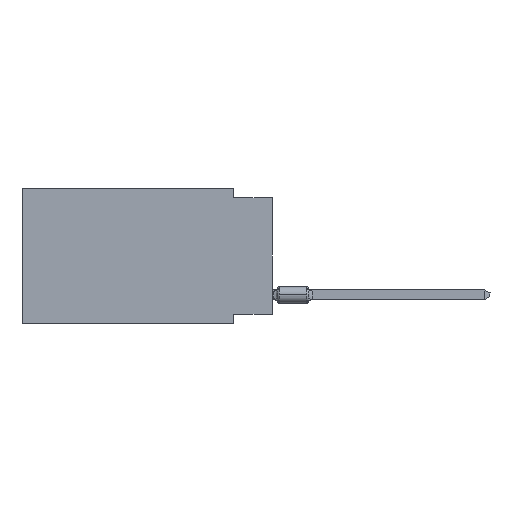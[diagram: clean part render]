
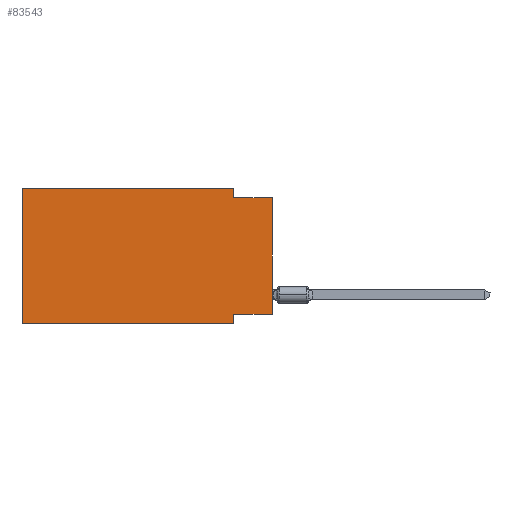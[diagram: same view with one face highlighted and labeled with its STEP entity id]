
A CAD part, left-side view. The second image highlights one B-rep face of the part: STEP entity #83543.
In plain terms, the highlighted planar face has unit normal (-1, 0, 0).
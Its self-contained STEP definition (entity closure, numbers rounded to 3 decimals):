
#1387 = FACE_OUTER_BOUND ( 'NONE', #75346, .T. ) ;
#3332 = DIRECTION ( 'NONE',  ( 0., 0., 1. ) ) ;
#4005 = ORIENTED_EDGE ( 'NONE', *, *, #35180, .F. ) ;
#4529 = CARTESIAN_POINT ( 'NONE',  ( 0., 2.54, -8.89 ) ) ;
#7326 = VERTEX_POINT ( 'NONE', #96517 ) ;
#8008 = CARTESIAN_POINT ( 'NONE',  ( 0., 2.54, -8.89 ) ) ;
#8583 = CARTESIAN_POINT ( 'NONE',  ( 0., 0., -8.255 ) ) ;
#10677 = DIRECTION ( 'NONE',  ( 0., -1., 0. ) ) ;
#14866 = VERTEX_POINT ( 'NONE', #88078 ) ;
#14873 = LINE ( 'NONE', #96654, #21799 ) ;
#15118 = ORIENTED_EDGE ( 'NONE', *, *, #36795, .T. ) ;
#15277 = VERTEX_POINT ( 'NONE', #24820 ) ;
#15380 = CARTESIAN_POINT ( 'NONE',  ( 0., 2.54, 0. ) ) ;
#17217 = DIRECTION ( 'NONE',  ( 0., -1., 0. ) ) ;
#20809 = CARTESIAN_POINT ( 'NONE',  ( 0., 0., -0.635 ) ) ;
#21293 = LINE ( 'NONE', #15380, #52518 ) ;
#21799 = VECTOR ( 'NONE', #104650, 1000. ) ;
#24820 = CARTESIAN_POINT ( 'NONE',  ( 0., 16.383, 0. ) ) ;
#25246 = VECTOR ( 'NONE', #25396, 1000. ) ;
#25396 = DIRECTION ( 'NONE',  ( 0., -1., 0. ) ) ;
#25451 = DIRECTION ( 'NONE',  ( 1., 0., 0. ) ) ;
#35180 = EDGE_CURVE ( 'NONE', #55034, #45108, #90320, .T. ) ;
#35359 = ORIENTED_EDGE ( 'NONE', *, *, #64687, .F. ) ;
#36795 = EDGE_CURVE ( 'NONE', #14866, #80378, #14873, .T. ) ;
#37780 = VECTOR ( 'NONE', #56697, 1000. ) ;
#40611 = DIRECTION ( 'NONE',  ( 0., 0., -1. ) ) ;
#40931 = ORIENTED_EDGE ( 'NONE', *, *, #84051, .F. ) ;
#41956 = LINE ( 'NONE', #49446, #25246 ) ;
#43768 = VECTOR ( 'NONE', #40611, 1000. ) ;
#43943 = LINE ( 'NONE', #76568, #55681 ) ;
#44126 = CARTESIAN_POINT ( 'NONE',  ( 0., 2.54, -8.255 ) ) ;
#44241 = ORIENTED_EDGE ( 'NONE', *, *, #94426, .F. ) ;
#44297 = VERTEX_POINT ( 'NONE', #101071 ) ;
#45108 = VERTEX_POINT ( 'NONE', #4529 ) ;
#46393 = DIRECTION ( 'NONE',  ( 0., 0., -1. ) ) ;
#49446 = CARTESIAN_POINT ( 'NONE',  ( 0., 16.383, -8.89 ) ) ;
#52518 = VECTOR ( 'NONE', #46393, 1000. ) ;
#55034 = VERTEX_POINT ( 'NONE', #44126 ) ;
#55681 = VECTOR ( 'NONE', #3332, 1000. ) ;
#56697 = DIRECTION ( 'NONE',  ( 0., 1., 0. ) ) ;
#58433 = VERTEX_POINT ( 'NONE', #75806 ) ;
#59618 = CARTESIAN_POINT ( 'NONE',  ( 0., 16.383, 0. ) ) ;
#64687 = EDGE_CURVE ( 'NONE', #58433, #80378, #105431, .T. ) ;
#66067 = DIRECTION ( 'NONE',  ( 0., 0., -1. ) ) ;
#66330 = EDGE_CURVE ( 'NONE', #7326, #15277, #43943, .T. ) ;
#75049 = ORIENTED_EDGE ( 'NONE', *, *, #87235, .F. ) ;
#75346 = EDGE_LOOP ( 'NONE', ( #15118, #35359, #44241, #75049, #80461, #102699, #4005, #40931 ) ) ;
#75806 = CARTESIAN_POINT ( 'NONE',  ( 0., 2.54, -0.635 ) ) ;
#76568 = CARTESIAN_POINT ( 'NONE',  ( 0., 16.383, 0. ) ) ;
#76965 = CARTESIAN_POINT ( 'NONE',  ( 0., 16.383, 0. ) ) ;
#77534 = VECTOR ( 'NONE', #10677, 1000. ) ;
#80378 = VERTEX_POINT ( 'NONE', #20809 ) ;
#80461 = ORIENTED_EDGE ( 'NONE', *, *, #66330, .F. ) ;
#83543 = ADVANCED_FACE ( 'NONE', ( #1387 ), #99728, .F. ) ;
#84051 = EDGE_CURVE ( 'NONE', #14866, #55034, #88273, .T. ) ;
#87235 = EDGE_CURVE ( 'NONE', #15277, #44297, #92994, .T. ) ;
#88078 = CARTESIAN_POINT ( 'NONE',  ( 0., 0., -8.255 ) ) ;
#88273 = LINE ( 'NONE', #8583, #37780 ) ;
#90320 = LINE ( 'NONE', #8008, #43768 ) ;
#92994 = LINE ( 'NONE', #76965, #77534 ) ;
#93264 = EDGE_CURVE ( 'NONE', #7326, #45108, #41956, .T. ) ;
#94426 = EDGE_CURVE ( 'NONE', #44297, #58433, #21293, .T. ) ;
#96517 = CARTESIAN_POINT ( 'NONE',  ( 0., 16.383, -8.89 ) ) ;
#96654 = CARTESIAN_POINT ( 'NONE',  ( 0., 0., 0. ) ) ;
#97425 = CARTESIAN_POINT ( 'NONE',  ( 0., 0., -0.635 ) ) ;
#99728 = PLANE ( 'NONE',  #104040 ) ;
#101071 = CARTESIAN_POINT ( 'NONE',  ( 0., 2.54, 0. ) ) ;
#102699 = ORIENTED_EDGE ( 'NONE', *, *, #93264, .T. ) ;
#103385 = VECTOR ( 'NONE', #17217, 1000. ) ;
#104040 = AXIS2_PLACEMENT_3D ( 'NONE', #59618, #25451, #66067 ) ;
#104650 = DIRECTION ( 'NONE',  ( 0., 0., 1. ) ) ;
#105431 = LINE ( 'NONE', #97425, #103385 ) ;
